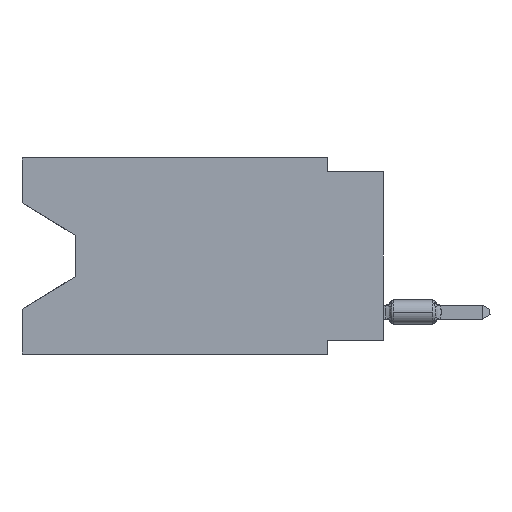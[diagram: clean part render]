
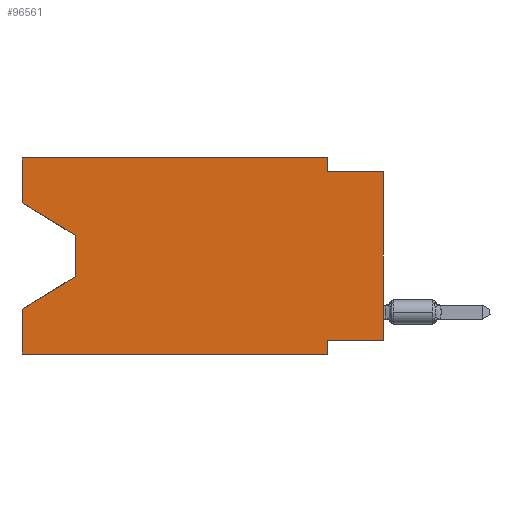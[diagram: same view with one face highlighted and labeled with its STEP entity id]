
A CAD part, left-side view. The second image highlights one B-rep face of the part: STEP entity #96561.
In plain terms, the highlighted planar face has unit normal (-1, 0, 0).
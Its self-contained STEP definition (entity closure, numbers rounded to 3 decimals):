
#44 = EDGE_CURVE ( 'NONE', #84567, #65714, #104248, .T. ) ;
#2711 = LINE ( 'NONE', #49667, #87655 ) ;
#2742 = CARTESIAN_POINT ( 'NONE',  ( 0., 2.54, -0.635 ) ) ;
#4261 = DIRECTION ( 'NONE',  ( 0., 0., -1. ) ) ;
#5667 = ORIENTED_EDGE ( 'NONE', *, *, #51344, .F. ) ;
#5740 = VERTEX_POINT ( 'NONE', #11362 ) ;
#6658 = CARTESIAN_POINT ( 'NONE',  ( 0., 0., -8.255 ) ) ;
#6893 = CARTESIAN_POINT ( 'NONE',  ( 0., 2.54, 0. ) ) ;
#7429 = VECTOR ( 'NONE', #54365, 1000. ) ;
#8495 = LINE ( 'NONE', #63870, #79000 ) ;
#9305 = CARTESIAN_POINT ( 'NONE',  ( 0., 0., 0. ) ) ;
#11362 = CARTESIAN_POINT ( 'NONE',  ( 0., 13.97, -5.385 ) ) ;
#11725 = DIRECTION ( 'NONE',  ( 0., -0.855, -0.519 ) ) ;
#12185 = CARTESIAN_POINT ( 'NONE',  ( 0., 13.97, -3.505 ) ) ;
#13434 = VECTOR ( 'NONE', #35596, 1000. ) ;
#14556 = EDGE_LOOP ( 'NONE', ( #23721, #68235, #78076, #30933, #57826, #5667, #98973, #50370, #34579, #32137, #40740, #16147 ) ) ;
#15048 = EDGE_CURVE ( 'NONE', #84763, #56595, #79852, .T. ) ;
#15504 = VECTOR ( 'NONE', #66549, 1000. ) ;
#16147 = ORIENTED_EDGE ( 'NONE', *, *, #15048, .F. ) ;
#17032 = LINE ( 'NONE', #58129, #15504 ) ;
#17592 = VERTEX_POINT ( 'NONE', #68872 ) ;
#19316 = CARTESIAN_POINT ( 'NONE',  ( 0., 16.383, -2.038 ) ) ;
#19612 = LINE ( 'NONE', #51816, #50266 ) ;
#19966 = DIRECTION ( 'NONE',  ( 0., 0., -1. ) ) ;
#20672 = VERTEX_POINT ( 'NONE', #77988 ) ;
#22466 = VERTEX_POINT ( 'NONE', #82369 ) ;
#23721 = ORIENTED_EDGE ( 'NONE', *, *, #40496, .T. ) ;
#24431 = EDGE_CURVE ( 'NONE', #20672, #71023, #52998, .T. ) ;
#28712 = CARTESIAN_POINT ( 'NONE',  ( 0., 2.54, 0. ) ) ;
#30933 = ORIENTED_EDGE ( 'NONE', *, *, #45747, .F. ) ;
#31388 = DIRECTION ( 'NONE',  ( 0., 0., 1. ) ) ;
#31767 = CARTESIAN_POINT ( 'NONE',  ( 0., 0., -0.635 ) ) ;
#32137 = ORIENTED_EDGE ( 'NONE', *, *, #44, .F. ) ;
#34579 = ORIENTED_EDGE ( 'NONE', *, *, #48633, .F. ) ;
#35596 = DIRECTION ( 'NONE',  ( 0., 0., -1. ) ) ;
#35699 = CARTESIAN_POINT ( 'NONE',  ( 0., 16.383, 0. ) ) ;
#37971 = LINE ( 'NONE', #12185, #78721 ) ;
#38203 = CARTESIAN_POINT ( 'NONE',  ( 0., 16.383, -8.89 ) ) ;
#40496 = EDGE_CURVE ( 'NONE', #84763, #22466, #19612, .T. ) ;
#40740 = ORIENTED_EDGE ( 'NONE', *, *, #52126, .F. ) ;
#43719 = FACE_OUTER_BOUND ( 'NONE', #14556, .T. ) ;
#45747 = EDGE_CURVE ( 'NONE', #20672, #17592, #2711, .T. ) ;
#47011 = DIRECTION ( 'NONE',  ( 0., 0.855, -0.519 ) ) ;
#48409 = AXIS2_PLACEMENT_3D ( 'NONE', #100566, #59504, #19966 ) ;
#48633 = EDGE_CURVE ( 'NONE', #65714, #88887, #17032, .T. ) ;
#49313 = CARTESIAN_POINT ( 'NONE',  ( 0., 16.383, 0. ) ) ;
#49667 = CARTESIAN_POINT ( 'NONE',  ( 0., 16.383, 0. ) ) ;
#50266 = VECTOR ( 'NONE', #11725, 1000. ) ;
#50370 = ORIENTED_EDGE ( 'NONE', *, *, #100479, .T. ) ;
#51344 = EDGE_CURVE ( 'NONE', #69955, #71023, #61741, .T. ) ;
#51816 = CARTESIAN_POINT ( 'NONE',  ( 0., 16.383, -2.038 ) ) ;
#51875 = VECTOR ( 'NONE', #31388, 1000. ) ;
#52067 = DIRECTION ( 'NONE',  ( 0., -1., 0. ) ) ;
#52126 = EDGE_CURVE ( 'NONE', #56595, #84567, #74683, .T. ) ;
#52408 = VECTOR ( 'NONE', #59357, 1000. ) ;
#52998 = LINE ( 'NONE', #38203, #56884 ) ;
#54365 = DIRECTION ( 'NONE',  ( 0., 0., -1. ) ) ;
#55162 = DIRECTION ( 'NONE',  ( 0., 1., 0. ) ) ;
#56595 = VERTEX_POINT ( 'NONE', #68637 ) ;
#56884 = VECTOR ( 'NONE', #86658, 1000. ) ;
#57826 = ORIENTED_EDGE ( 'NONE', *, *, #24431, .T. ) ;
#58129 = CARTESIAN_POINT ( 'NONE',  ( 0., 0., -0.635 ) ) ;
#59357 = DIRECTION ( 'NONE',  ( 0., 0., 1. ) ) ;
#59504 = DIRECTION ( 'NONE',  ( 1., 0., 0. ) ) ;
#61741 = LINE ( 'NONE', #71699, #7429 ) ;
#63870 = CARTESIAN_POINT ( 'NONE',  ( 0., 13.97, -5.385 ) ) ;
#65060 = EDGE_CURVE ( 'NONE', #100516, #69955, #93092, .T. ) ;
#65714 = VERTEX_POINT ( 'NONE', #2742 ) ;
#65724 = LINE ( 'NONE', #9305, #52408 ) ;
#66549 = DIRECTION ( 'NONE',  ( 0., -1., 0. ) ) ;
#68235 = ORIENTED_EDGE ( 'NONE', *, *, #94671, .T. ) ;
#68637 = CARTESIAN_POINT ( 'NONE',  ( 0., 16.383, 0. ) ) ;
#68872 = CARTESIAN_POINT ( 'NONE',  ( 0., 16.383, -6.852 ) ) ;
#69955 = VERTEX_POINT ( 'NONE', #83110 ) ;
#71023 = VERTEX_POINT ( 'NONE', #77457 ) ;
#71525 = VECTOR ( 'NONE', #52067, 1000. ) ;
#71699 = CARTESIAN_POINT ( 'NONE',  ( 0., 2.54, -8.89 ) ) ;
#74683 = LINE ( 'NONE', #35699, #71525 ) ;
#77457 = CARTESIAN_POINT ( 'NONE',  ( 0., 2.54, -8.89 ) ) ;
#77988 = CARTESIAN_POINT ( 'NONE',  ( 0., 16.383, -8.89 ) ) ;
#78076 = ORIENTED_EDGE ( 'NONE', *, *, #87084, .T. ) ;
#78721 = VECTOR ( 'NONE', #4261, 1000. ) ;
#79000 = VECTOR ( 'NONE', #47011, 1000. ) ;
#79852 = LINE ( 'NONE', #49313, #51875 ) ;
#81787 = DIRECTION ( 'NONE',  ( 0., 0., 1. ) ) ;
#82369 = CARTESIAN_POINT ( 'NONE',  ( 0., 13.97, -3.505 ) ) ;
#83110 = CARTESIAN_POINT ( 'NONE',  ( 0., 2.54, -8.255 ) ) ;
#84567 = VERTEX_POINT ( 'NONE', #6893 ) ;
#84763 = VERTEX_POINT ( 'NONE', #19316 ) ;
#86658 = DIRECTION ( 'NONE',  ( 0., -1., 0. ) ) ;
#87084 = EDGE_CURVE ( 'NONE', #5740, #17592, #8495, .T. ) ;
#87655 = VECTOR ( 'NONE', #81787, 1000. ) ;
#88887 = VERTEX_POINT ( 'NONE', #31767 ) ;
#92160 = PLANE ( 'NONE',  #48409 ) ;
#93092 = LINE ( 'NONE', #6658, #94839 ) ;
#94671 = EDGE_CURVE ( 'NONE', #22466, #5740, #37971, .T. ) ;
#94839 = VECTOR ( 'NONE', #55162, 1000. ) ;
#96561 = ADVANCED_FACE ( 'NONE', ( #43719 ), #92160, .F. ) ;
#97815 = CARTESIAN_POINT ( 'NONE',  ( 0., 0., -8.255 ) ) ;
#98973 = ORIENTED_EDGE ( 'NONE', *, *, #65060, .F. ) ;
#100479 = EDGE_CURVE ( 'NONE', #100516, #88887, #65724, .T. ) ;
#100516 = VERTEX_POINT ( 'NONE', #97815 ) ;
#100566 = CARTESIAN_POINT ( 'NONE',  ( 0., 16.383, 0. ) ) ;
#104248 = LINE ( 'NONE', #28712, #13434 ) ;
